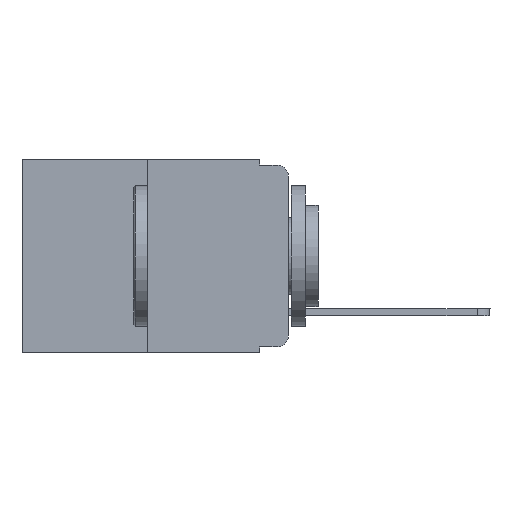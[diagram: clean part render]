
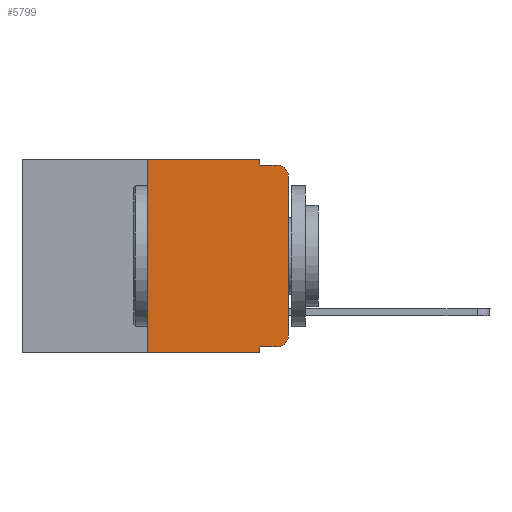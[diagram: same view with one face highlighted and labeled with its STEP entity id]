
A CAD part, left-side view. The second image highlights one B-rep face of the part: STEP entity #5799.
In plain terms, the highlighted planar face has unit normal (-1, 0, 0).
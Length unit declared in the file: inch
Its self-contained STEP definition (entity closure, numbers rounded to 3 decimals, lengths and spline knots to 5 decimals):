
#78 = ORIENTED_EDGE ( 'NONE', *, *, #8247, .T. ) ;
#322 = DIRECTION ( 'NONE',  ( 0., 0., -1. ) ) ;
#382 = DIRECTION ( 'NONE',  ( -1., 0., 0. ) ) ;
#600 = CARTESIAN_POINT ( 'NONE',  ( 0., 0.051, -0.333 ) ) ;
#636 = PLANE ( 'NONE',  #9045 ) ;
#716 = VERTEX_POINT ( 'NONE', #7262 ) ;
#812 = VECTOR ( 'NONE', #11307, 39.37008 ) ;
#851 = DIRECTION ( 'NONE',  ( 0., -1., 0. ) ) ;
#1030 = CARTESIAN_POINT ( 'NONE',  ( 0., 0., 0. ) ) ;
#1215 = EDGE_CURVE ( 'NONE', #8797, #8966, #7529, .T. ) ;
#1291 = EDGE_CURVE ( 'NONE', #5764, #716, #4836, .T. ) ;
#1400 = CARTESIAN_POINT ( 'NONE',  ( 0., 0., -0.313 ) ) ;
#1457 = VERTEX_POINT ( 'NONE', #1400 ) ;
#1750 = CARTESIAN_POINT ( 'NONE',  ( 0., 0.473, 0. ) ) ;
#1759 = VECTOR ( 'NONE', #5874, 39.37008 ) ;
#1895 = CARTESIAN_POINT ( 'NONE',  ( 0., 0.051, 0. ) ) ;
#2084 = VERTEX_POINT ( 'NONE', #9562 ) ;
#2086 = CIRCLE ( 'NONE', #4633, 0.02 ) ;
#2384 = ORIENTED_EDGE ( 'NONE', *, *, #1215, .F. ) ;
#2401 = EDGE_CURVE ( 'NONE', #8267, #10793, #9201, .T. ) ;
#2557 = LINE ( 'NONE', #12074, #3814 ) ;
#2611 = CARTESIAN_POINT ( 'NONE',  ( 0., 0.051, -0.01 ) ) ;
#2685 = DIRECTION ( 'NONE',  ( 0., -1., 0. ) ) ;
#2746 = ORIENTED_EDGE ( 'NONE', *, *, #9238, .T. ) ;
#2811 = VECTOR ( 'NONE', #11226, 39.37008 ) ;
#3120 = LINE ( 'NONE', #6773, #1759 ) ;
#3272 = CARTESIAN_POINT ( 'NONE',  ( 0., 0.02, -0.313 ) ) ;
#3814 = VECTOR ( 'NONE', #2685, 39.37008 ) ;
#3896 = EDGE_LOOP ( 'NONE', ( #10078, #10521, #4735, #5071, #5042, #2384, #2746, #8657, #5501, #78 ) ) ;
#4172 = CARTESIAN_POINT ( 'NONE',  ( 0., 0.051, -0.343 ) ) ;
#4506 = DIRECTION ( 'NONE',  ( 1., 0., 0. ) ) ;
#4561 = CARTESIAN_POINT ( 'NONE',  ( 0., 0.473, 0. ) ) ;
#4633 = AXIS2_PLACEMENT_3D ( 'NONE', #10438, #4907, #9507 ) ;
#4670 = EDGE_CURVE ( 'NONE', #2084, #716, #2086, .T. ) ;
#4735 = ORIENTED_EDGE ( 'NONE', *, *, #1291, .F. ) ;
#4836 = LINE ( 'NONE', #10364, #7648 ) ;
#4864 = CARTESIAN_POINT ( 'NONE',  ( 0., 0.051, 0. ) ) ;
#4907 = DIRECTION ( 'NONE',  ( -1., 0., 0. ) ) ;
#5042 = ORIENTED_EDGE ( 'NONE', *, *, #9758, .F. ) ;
#5071 = ORIENTED_EDGE ( 'NONE', *, *, #7349, .F. ) ;
#5488 = DIRECTION ( 'NONE',  ( 0., 0., -1. ) ) ;
#5501 = ORIENTED_EDGE ( 'NONE', *, *, #2401, .T. ) ;
#5505 = EDGE_CURVE ( 'NONE', #1457, #2084, #9368, .T. ) ;
#5514 = CARTESIAN_POINT ( 'NONE',  ( 0., 0.25, 0. ) ) ;
#5764 = VERTEX_POINT ( 'NONE', #2611 ) ;
#5799 = ADVANCED_FACE ( 'NONE', ( #8995 ), #636, .F. ) ;
#5874 = DIRECTION ( 'NONE',  ( 0., 0., -1. ) ) ;
#6233 = CARTESIAN_POINT ( 'NONE',  ( 0., 0.25, -0.343 ) ) ;
#6773 = CARTESIAN_POINT ( 'NONE',  ( 0., 0.051, 0. ) ) ;
#6992 = VERTEX_POINT ( 'NONE', #4172 ) ;
#7066 = AXIS2_PLACEMENT_3D ( 'NONE', #3272, #382, #322 ) ;
#7262 = CARTESIAN_POINT ( 'NONE',  ( 0., 0.02, -0.01 ) ) ;
#7349 = EDGE_CURVE ( 'NONE', #9407, #5764, #3120, .T. ) ;
#7464 = LINE ( 'NONE', #1895, #11900 ) ;
#7529 = LINE ( 'NONE', #10489, #812 ) ;
#7648 = VECTOR ( 'NONE', #9325, 39.37008 ) ;
#7828 = VECTOR ( 'NONE', #12002, 39.37008 ) ;
#8247 = EDGE_CURVE ( 'NONE', #10793, #1457, #8397, .T. ) ;
#8267 = VERTEX_POINT ( 'NONE', #11637 ) ;
#8397 = CIRCLE ( 'NONE', #7066, 0.02 ) ;
#8657 = ORIENTED_EDGE ( 'NONE', *, *, #8920, .F. ) ;
#8797 = VERTEX_POINT ( 'NONE', #6233 ) ;
#8828 = VECTOR ( 'NONE', #851, 39.37008 ) ;
#8920 = EDGE_CURVE ( 'NONE', #8267, #6992, #7464, .T. ) ;
#8966 = VERTEX_POINT ( 'NONE', #5514 ) ;
#8995 = FACE_OUTER_BOUND ( 'NONE', #3896, .T. ) ;
#9045 = AXIS2_PLACEMENT_3D ( 'NONE', #1750, #4506, #5488 ) ;
#9073 = DIRECTION ( 'NONE',  ( 0., 0., -1. ) ) ;
#9201 = LINE ( 'NONE', #600, #8828 ) ;
#9238 = EDGE_CURVE ( 'NONE', #8797, #6992, #2557, .T. ) ;
#9325 = DIRECTION ( 'NONE',  ( 0., -1., 0. ) ) ;
#9368 = LINE ( 'NONE', #1030, #2811 ) ;
#9407 = VERTEX_POINT ( 'NONE', #4864 ) ;
#9507 = DIRECTION ( 'NONE',  ( 0., 0., -1. ) ) ;
#9562 = CARTESIAN_POINT ( 'NONE',  ( 0., 0., -0.03 ) ) ;
#9758 = EDGE_CURVE ( 'NONE', #8966, #9407, #11873, .T. ) ;
#10078 = ORIENTED_EDGE ( 'NONE', *, *, #5505, .T. ) ;
#10364 = CARTESIAN_POINT ( 'NONE',  ( 0., 0.051, -0.01 ) ) ;
#10438 = CARTESIAN_POINT ( 'NONE',  ( 0., 0.02, -0.03 ) ) ;
#10489 = CARTESIAN_POINT ( 'NONE',  ( 0., 0.25, 0. ) ) ;
#10521 = ORIENTED_EDGE ( 'NONE', *, *, #4670, .T. ) ;
#10793 = VERTEX_POINT ( 'NONE', #11299 ) ;
#11226 = DIRECTION ( 'NONE',  ( 0., 0., 1. ) ) ;
#11299 = CARTESIAN_POINT ( 'NONE',  ( 0., 0.02, -0.333 ) ) ;
#11307 = DIRECTION ( 'NONE',  ( 0., 0., 1. ) ) ;
#11637 = CARTESIAN_POINT ( 'NONE',  ( 0., 0.051, -0.333 ) ) ;
#11873 = LINE ( 'NONE', #4561, #7828 ) ;
#11900 = VECTOR ( 'NONE', #9073, 39.37008 ) ;
#12002 = DIRECTION ( 'NONE',  ( 0., -1., 0. ) ) ;
#12074 = CARTESIAN_POINT ( 'NONE',  ( 0., 0.473, -0.343 ) ) ;
